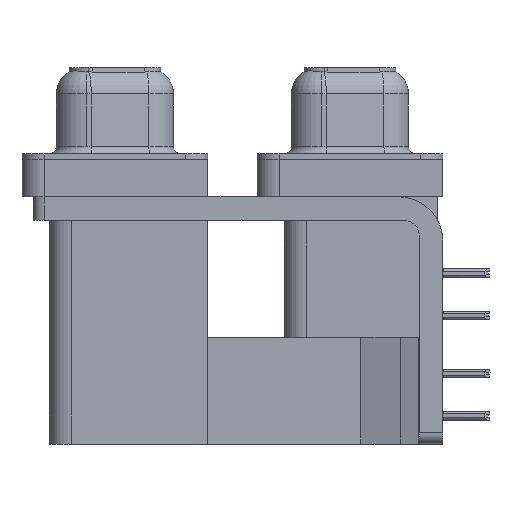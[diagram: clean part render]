
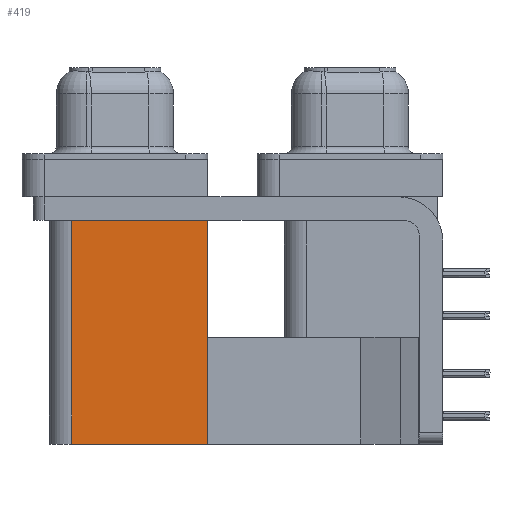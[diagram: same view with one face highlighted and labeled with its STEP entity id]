
A CAD part, left-side view. The second image highlights one B-rep face of the part: STEP entity #419.
In plain terms, the highlighted planar face has unit normal (-1, 0, 0).
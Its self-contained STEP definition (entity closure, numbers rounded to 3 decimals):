
#419 = ADVANCED_FACE ( 'NONE', ( #4283 ), #23215, .F. ) ;
#448 = LINE ( 'NONE', #1308, #29844 ) ;
#826 = VECTOR ( 'NONE', #28207, 1000. ) ;
#1308 = CARTESIAN_POINT ( 'NONE',  ( 3.79, 9.6, -19.2 ) ) ;
#2881 = CARTESIAN_POINT ( 'NONE',  ( 3.79, 9.6, -19.2 ) ) ;
#4249 = ORIENTED_EDGE ( 'NONE', *, *, #20655, .F. ) ;
#4283 = FACE_OUTER_BOUND ( 'NONE', #35507, .T. ) ;
#4702 = CARTESIAN_POINT ( 'NONE',  ( 3.79, 9.6, -19.2 ) ) ;
#7629 = LINE ( 'NONE', #18215, #826 ) ;
#7957 = EDGE_CURVE ( 'NONE', #18722, #24298, #7629, .T. ) ;
#8682 = AXIS2_PLACEMENT_3D ( 'NONE', #4702, #33612, #33180 ) ;
#10840 = CARTESIAN_POINT ( 'NONE',  ( 3.79, 18.8, -2.5 ) ) ;
#12183 = ORIENTED_EDGE ( 'NONE', *, *, #25923, .T. ) ;
#14192 = DIRECTION ( 'NONE',  ( 0., 0., 1. ) ) ;
#15689 = DIRECTION ( 'NONE',  ( 0., 0., 1. ) ) ;
#17451 = LINE ( 'NONE', #2881, #20055 ) ;
#18215 = CARTESIAN_POINT ( 'NONE',  ( 3.79, 9.6, -2.5 ) ) ;
#18722 = VERTEX_POINT ( 'NONE', #31465 ) ;
#19269 = VERTEX_POINT ( 'NONE', #41980 ) ;
#20055 = VECTOR ( 'NONE', #15689, 1000. ) ;
#20655 = EDGE_CURVE ( 'NONE', #19269, #24298, #37342, .T. ) ;
#23215 = PLANE ( 'NONE',  #8682 ) ;
#24298 = VERTEX_POINT ( 'NONE', #10840 ) ;
#24760 = CARTESIAN_POINT ( 'NONE',  ( 3.79, 9.6, -19.2 ) ) ;
#25923 = EDGE_CURVE ( 'NONE', #26213, #18722, #17451, .T. ) ;
#26213 = VERTEX_POINT ( 'NONE', #24760 ) ;
#28207 = DIRECTION ( 'NONE',  ( 0., 1., 0. ) ) ;
#29844 = VECTOR ( 'NONE', #32778, 1000. ) ;
#31465 = CARTESIAN_POINT ( 'NONE',  ( 3.79, 9.6, -2.5 ) ) ;
#32223 = ORIENTED_EDGE ( 'NONE', *, *, #34241, .F. ) ;
#32778 = DIRECTION ( 'NONE',  ( 0., 1., 0. ) ) ;
#33180 = DIRECTION ( 'NONE',  ( 0., 1., 0. ) ) ;
#33612 = DIRECTION ( 'NONE',  ( 1., 0., 0. ) ) ;
#33939 = CARTESIAN_POINT ( 'NONE',  ( 3.79, 18.8, -19.2 ) ) ;
#34241 = EDGE_CURVE ( 'NONE', #26213, #19269, #448, .T. ) ;
#35507 = EDGE_LOOP ( 'NONE', ( #37499, #4249, #32223, #12183 ) ) ;
#37342 = LINE ( 'NONE', #33939, #39417 ) ;
#37499 = ORIENTED_EDGE ( 'NONE', *, *, #7957, .T. ) ;
#39417 = VECTOR ( 'NONE', #14192, 1000. ) ;
#41980 = CARTESIAN_POINT ( 'NONE',  ( 3.79, 18.8, -19.2 ) ) ;
